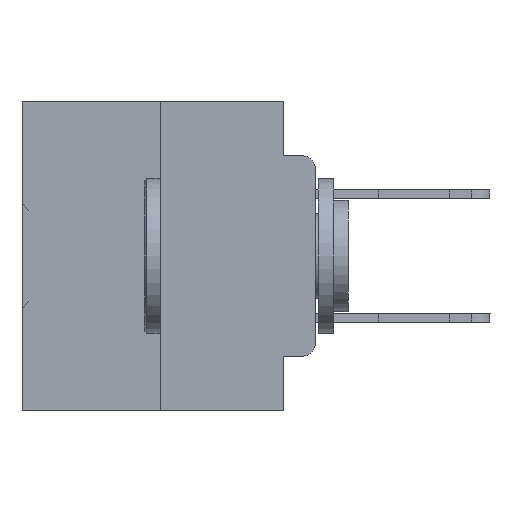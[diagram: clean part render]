
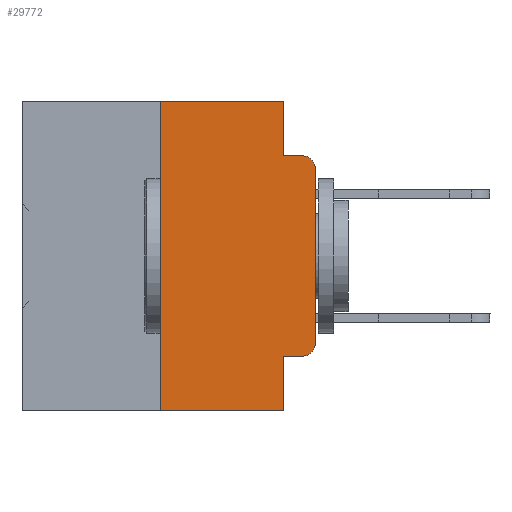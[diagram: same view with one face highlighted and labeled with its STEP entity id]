
A CAD part, left-side view. The second image highlights one B-rep face of the part: STEP entity #29772.
In plain terms, the highlighted planar face has unit normal (-1, 0, 0).
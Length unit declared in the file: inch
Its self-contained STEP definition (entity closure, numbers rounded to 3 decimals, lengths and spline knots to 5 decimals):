
#723 = EDGE_CURVE ( 'NONE', #8486, #3634, #15479, .T. ) ;
#1038 = EDGE_CURVE ( 'NONE', #39879, #1438, #33339, .T. ) ;
#1438 = VERTEX_POINT ( 'NONE', #34681 ) ;
#1587 = EDGE_CURVE ( 'NONE', #25602, #23249, #27970, .T. ) ;
#1622 = ORIENTED_EDGE ( 'NONE', *, *, #27516, .T. ) ;
#2921 = VECTOR ( 'NONE', #20245, 39.37008 ) ;
#3634 = VERTEX_POINT ( 'NONE', #5616 ) ;
#3914 = DIRECTION ( 'NONE',  ( 0., 0., -1. ) ) ;
#4041 = ORIENTED_EDGE ( 'NONE', *, *, #1587, .T. ) ;
#4089 = ORIENTED_EDGE ( 'NONE', *, *, #8832, .F. ) ;
#4731 = CARTESIAN_POINT ( 'NONE',  ( 0., 0.473, 0. ) ) ;
#5049 = CARTESIAN_POINT ( 'NONE',  ( 0., 0.051, -0.0885 ) ) ;
#5616 = CARTESIAN_POINT ( 'NONE',  ( 0., 0.051, -0.5 ) ) ;
#6317 = CARTESIAN_POINT ( 'NONE',  ( 0., 0.25, -0.5 ) ) ;
#6387 = FACE_OUTER_BOUND ( 'NONE', #31957, .T. ) ;
#6487 = CARTESIAN_POINT ( 'NONE',  ( 0., 0.02, -0.0885 ) ) ;
#6716 = CARTESIAN_POINT ( 'NONE',  ( 0., 0.25, 0. ) ) ;
#6833 = DIRECTION ( 'NONE',  ( 0., 0., 1. ) ) ;
#6850 = LINE ( 'NONE', #15785, #18042 ) ;
#7119 = AXIS2_PLACEMENT_3D ( 'NONE', #38220, #16943, #13962 ) ;
#7357 = PLANE ( 'NONE',  #7119 ) ;
#8486 = VERTEX_POINT ( 'NONE', #6317 ) ;
#8832 = EDGE_CURVE ( 'NONE', #34127, #3634, #9012, .T. ) ;
#9012 = LINE ( 'NONE', #9055, #22980 ) ;
#9055 = CARTESIAN_POINT ( 'NONE',  ( 0., 0.051, 0. ) ) ;
#9429 = DIRECTION ( 'NONE',  ( 0., 0., -1. ) ) ;
#9987 = VERTEX_POINT ( 'NONE', #6487 ) ;
#10893 = EDGE_CURVE ( 'NONE', #8486, #39879, #21885, .T. ) ;
#11237 = EDGE_CURVE ( 'NONE', #1438, #31926, #6850, .T. ) ;
#11908 = EDGE_CURVE ( 'NONE', #31926, #9987, #19377, .T. ) ;
#12251 = VECTOR ( 'NONE', #19975, 39.37008 ) ;
#12593 = VECTOR ( 'NONE', #38687, 39.37008 ) ;
#12607 = DIRECTION ( 'NONE',  ( 0., 0., -1. ) ) ;
#12653 = ORIENTED_EDGE ( 'NONE', *, *, #723, .T. ) ;
#13585 = CIRCLE ( 'NONE', #15825, 0.02 ) ;
#13629 = VECTOR ( 'NONE', #26774, 39.37008 ) ;
#13962 = DIRECTION ( 'NONE',  ( 0., 0., -1. ) ) ;
#15479 = LINE ( 'NONE', #16744, #33795 ) ;
#15785 = CARTESIAN_POINT ( 'NONE',  ( 0., 0.051, 0. ) ) ;
#15825 = AXIS2_PLACEMENT_3D ( 'NONE', #25280, #31117, #12607 ) ;
#16744 = CARTESIAN_POINT ( 'NONE',  ( 0., 0.473, -0.5 ) ) ;
#16927 = CARTESIAN_POINT ( 'NONE',  ( 0., 0.02, -0.4115 ) ) ;
#16943 = DIRECTION ( 'NONE',  ( 1., 0., 0. ) ) ;
#17341 = CARTESIAN_POINT ( 'NONE',  ( 0., 0.051, -0.4115 ) ) ;
#17813 = EDGE_CURVE ( 'NONE', #34127, #33117, #32530, .T. ) ;
#18042 = VECTOR ( 'NONE', #3914, 39.37008 ) ;
#18257 = CIRCLE ( 'NONE', #21408, 0.02 ) ;
#18366 = DIRECTION ( 'NONE',  ( 0., 0., -1. ) ) ;
#18576 = ORIENTED_EDGE ( 'NONE', *, *, #35069, .T. ) ;
#19377 = LINE ( 'NONE', #35744, #12593 ) ;
#19975 = DIRECTION ( 'NONE',  ( 0., -1., 0. ) ) ;
#20245 = DIRECTION ( 'NONE',  ( 0., -1., 0. ) ) ;
#21408 = AXIS2_PLACEMENT_3D ( 'NONE', #27508, #30617, #9429 ) ;
#21885 = LINE ( 'NONE', #23685, #13629 ) ;
#22980 = VECTOR ( 'NONE', #18366, 39.37008 ) ;
#23084 = ORIENTED_EDGE ( 'NONE', *, *, #11908, .F. ) ;
#23249 = VERTEX_POINT ( 'NONE', #23674 ) ;
#23674 = CARTESIAN_POINT ( 'NONE',  ( 0., 0., -0.1085 ) ) ;
#23685 = CARTESIAN_POINT ( 'NONE',  ( 0., 0.25, 0. ) ) ;
#24550 = ORIENTED_EDGE ( 'NONE', *, *, #10893, .F. ) ;
#25142 = ORIENTED_EDGE ( 'NONE', *, *, #11237, .F. ) ;
#25280 = CARTESIAN_POINT ( 'NONE',  ( 0., 0.02, -0.1085 ) ) ;
#25602 = VERTEX_POINT ( 'NONE', #27349 ) ;
#26774 = DIRECTION ( 'NONE',  ( 0., 0., 1. ) ) ;
#27349 = CARTESIAN_POINT ( 'NONE',  ( 0., 0., -0.3915 ) ) ;
#27508 = CARTESIAN_POINT ( 'NONE',  ( 0., 0.02, -0.3915 ) ) ;
#27516 = EDGE_CURVE ( 'NONE', #33117, #25602, #18257, .T. ) ;
#27970 = LINE ( 'NONE', #37219, #29466 ) ;
#29466 = VECTOR ( 'NONE', #6833, 39.37008 ) ;
#29772 = ADVANCED_FACE ( 'NONE', ( #6387 ), #7357, .F. ) ;
#30617 = DIRECTION ( 'NONE',  ( -1., 0., 0. ) ) ;
#31117 = DIRECTION ( 'NONE',  ( -1., 0., 0. ) ) ;
#31926 = VERTEX_POINT ( 'NONE', #5049 ) ;
#31957 = EDGE_LOOP ( 'NONE', ( #4041, #18576, #23084, #25142, #34188, #24550, #12653, #4089, #36804, #1622 ) ) ;
#32238 = CARTESIAN_POINT ( 'NONE',  ( 0., 0.051, -0.4115 ) ) ;
#32530 = LINE ( 'NONE', #32238, #12251 ) ;
#33117 = VERTEX_POINT ( 'NONE', #16927 ) ;
#33339 = LINE ( 'NONE', #4731, #2921 ) ;
#33795 = VECTOR ( 'NONE', #38570, 39.37008 ) ;
#34127 = VERTEX_POINT ( 'NONE', #17341 ) ;
#34188 = ORIENTED_EDGE ( 'NONE', *, *, #1038, .F. ) ;
#34681 = CARTESIAN_POINT ( 'NONE',  ( 0., 0.051, 0. ) ) ;
#35069 = EDGE_CURVE ( 'NONE', #23249, #9987, #13585, .T. ) ;
#35744 = CARTESIAN_POINT ( 'NONE',  ( 0., 0.051, -0.0885 ) ) ;
#36804 = ORIENTED_EDGE ( 'NONE', *, *, #17813, .T. ) ;
#37219 = CARTESIAN_POINT ( 'NONE',  ( 0., 0., 0. ) ) ;
#38220 = CARTESIAN_POINT ( 'NONE',  ( 0., 0.473, 0. ) ) ;
#38570 = DIRECTION ( 'NONE',  ( 0., -1., 0. ) ) ;
#38687 = DIRECTION ( 'NONE',  ( 0., -1., 0. ) ) ;
#39879 = VERTEX_POINT ( 'NONE', #6716 ) ;
